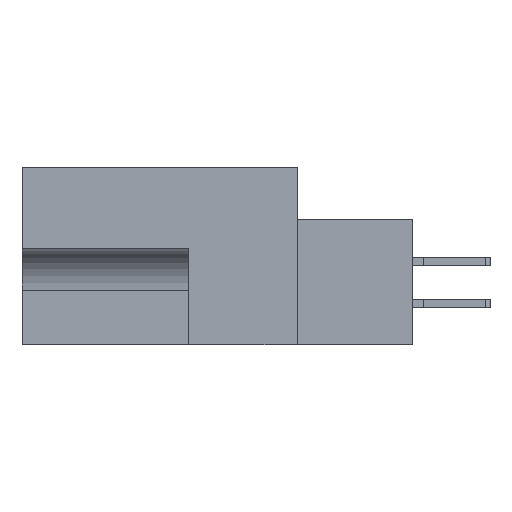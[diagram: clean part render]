
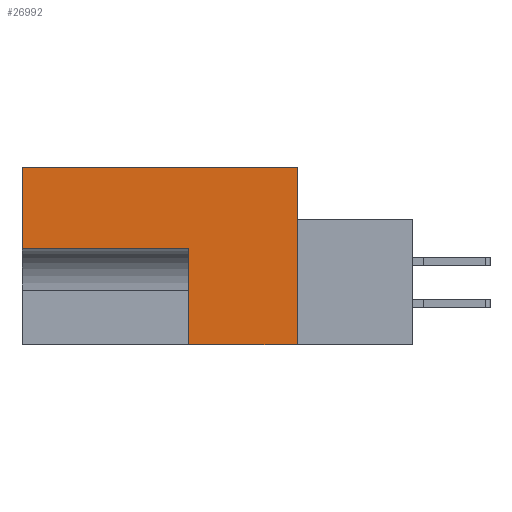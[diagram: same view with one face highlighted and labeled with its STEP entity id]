
A CAD part, left-side view. The second image highlights one B-rep face of the part: STEP entity #26992.
In plain terms, the highlighted planar face has unit normal (-1, 0, 0).
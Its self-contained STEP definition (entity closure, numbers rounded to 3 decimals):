
#27 = VERTEX_POINT ( 'NONE', #6574 ) ;
#694 = LINE ( 'NONE', #11963, #29732 ) ;
#2209 = VERTEX_POINT ( 'NONE', #13288 ) ;
#3704 = CARTESIAN_POINT ( 'NONE',  ( 0., 8.255, -6.172 ) ) ;
#3822 = DIRECTION ( 'NONE',  ( 0., 1., 0. ) ) ;
#3966 = ORIENTED_EDGE ( 'NONE', *, *, #6302, .F. ) ;
#4464 = DIRECTION ( 'NONE',  ( 0., 0., -1. ) ) ;
#5143 = LINE ( 'NONE', #28432, #8113 ) ;
#5214 = VECTOR ( 'NONE', #25664, 1000. ) ;
#5716 = CARTESIAN_POINT ( 'NONE',  ( 0., 0., -13.487 ) ) ;
#5885 = AXIS2_PLACEMENT_3D ( 'NONE', #34481, #15299, #4464 ) ;
#5960 = ORIENTED_EDGE ( 'NONE', *, *, #16407, .F. ) ;
#6302 = EDGE_CURVE ( 'NONE', #27, #11061, #694, .T. ) ;
#6574 = CARTESIAN_POINT ( 'NONE',  ( 0., 8.255, -13.487 ) ) ;
#6636 = FACE_OUTER_BOUND ( 'NONE', #9177, .T. ) ;
#6940 = PLANE ( 'NONE',  #5885 ) ;
#7120 = EDGE_CURVE ( 'NONE', #24753, #27, #12561, .T. ) ;
#7586 = DIRECTION ( 'NONE',  ( 0., 1., 0. ) ) ;
#8113 = VECTOR ( 'NONE', #32089, 1000. ) ;
#8356 = LINE ( 'NONE', #24419, #31797 ) ;
#9177 = EDGE_LOOP ( 'NONE', ( #16290, #32643, #5960, #20901, #10420, #3966 ) ) ;
#9700 = EDGE_CURVE ( 'NONE', #2209, #15570, #5143, .T. ) ;
#10420 = ORIENTED_EDGE ( 'NONE', *, *, #13162, .F. ) ;
#11061 = VERTEX_POINT ( 'NONE', #14349 ) ;
#11963 = CARTESIAN_POINT ( 'NONE',  ( 0., 8.255, -13.487 ) ) ;
#12561 = LINE ( 'NONE', #27288, #27106 ) ;
#13162 = EDGE_CURVE ( 'NONE', #11061, #2209, #17503, .T. ) ;
#13288 = CARTESIAN_POINT ( 'NONE',  ( 0., 20.955, -6.172 ) ) ;
#14349 = CARTESIAN_POINT ( 'NONE',  ( 0., 8.255, -6.172 ) ) ;
#15299 = DIRECTION ( 'NONE',  ( 1., 0., 0. ) ) ;
#15570 = VERTEX_POINT ( 'NONE', #20198 ) ;
#16290 = ORIENTED_EDGE ( 'NONE', *, *, #7120, .F. ) ;
#16407 = EDGE_CURVE ( 'NONE', #15570, #35276, #8356, .T. ) ;
#17503 = LINE ( 'NONE', #3704, #20064 ) ;
#18965 = EDGE_CURVE ( 'NONE', #35276, #24753, #31675, .T. ) ;
#20064 = VECTOR ( 'NONE', #3822, 1000. ) ;
#20198 = CARTESIAN_POINT ( 'NONE',  ( 0., 20.955, 0. ) ) ;
#20901 = ORIENTED_EDGE ( 'NONE', *, *, #9700, .F. ) ;
#22529 = CARTESIAN_POINT ( 'NONE',  ( 0., 0., 0. ) ) ;
#24419 = CARTESIAN_POINT ( 'NONE',  ( 0., 11.506, 0. ) ) ;
#24753 = VERTEX_POINT ( 'NONE', #5716 ) ;
#25664 = DIRECTION ( 'NONE',  ( 0., 0., -1. ) ) ;
#26992 = ADVANCED_FACE ( 'NONE', ( #6636 ), #6940, .F. ) ;
#27106 = VECTOR ( 'NONE', #7586, 1000. ) ;
#27288 = CARTESIAN_POINT ( 'NONE',  ( 0., -8.814, -13.487 ) ) ;
#28432 = CARTESIAN_POINT ( 'NONE',  ( 0., 20.955, -13.487 ) ) ;
#29732 = VECTOR ( 'NONE', #31198, 1000. ) ;
#31198 = DIRECTION ( 'NONE',  ( 0., 0., 1. ) ) ;
#31675 = LINE ( 'NONE', #33650, #5214 ) ;
#31797 = VECTOR ( 'NONE', #32772, 1000. ) ;
#32089 = DIRECTION ( 'NONE',  ( 0., 0., 1. ) ) ;
#32643 = ORIENTED_EDGE ( 'NONE', *, *, #18965, .F. ) ;
#32772 = DIRECTION ( 'NONE',  ( 0., -1., 0. ) ) ;
#33650 = CARTESIAN_POINT ( 'NONE',  ( 0., 0., 0. ) ) ;
#34481 = CARTESIAN_POINT ( 'NONE',  ( 0., 0., 0. ) ) ;
#35276 = VERTEX_POINT ( 'NONE', #22529 ) ;
